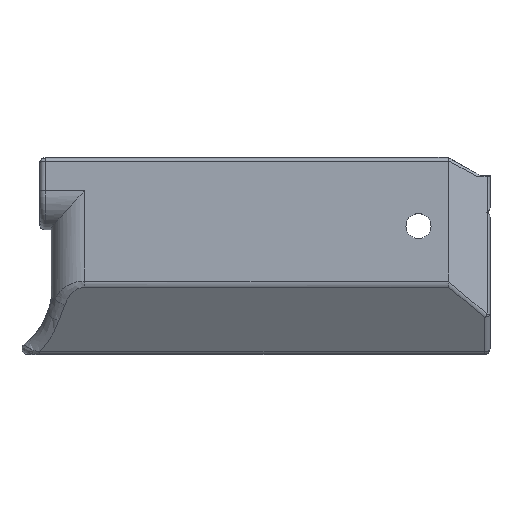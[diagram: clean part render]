
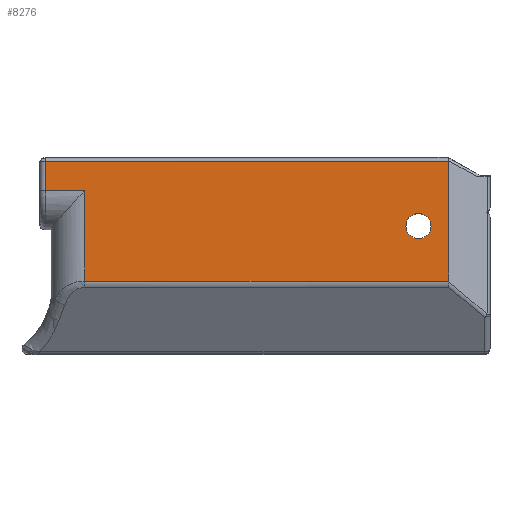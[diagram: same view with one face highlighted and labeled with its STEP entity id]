
A CAD part, top view. The second image highlights one B-rep face of the part: STEP entity #8276.
In plain terms, the highlighted planar face has unit normal (0, 0, 1).
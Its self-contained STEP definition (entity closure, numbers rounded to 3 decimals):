
#42=FACE_BOUND('',#2025,.T.);
#1062=PLANE('',#8491);
#1556=FACE_OUTER_BOUND('',#2024,.T.);
#2024=EDGE_LOOP('',(#7696,#7697,#7698,#7699,#7700,#7701));
#2025=EDGE_LOOP('',(#7702));
#2065=LINE('',#9587,#2628);
#2071=LINE('',#9659,#2634);
#2587=LINE('',#16405,#3150);
#2588=LINE('',#16408,#3151);
#2589=LINE('',#16409,#3152);
#2590=LINE('',#16410,#3153);
#2628=VECTOR('',#8560,10.);
#2634=VECTOR('',#8594,10.);
#3150=VECTOR('',#9428,10.);
#3151=VECTOR('',#9431,7.);
#3152=VECTOR('',#9432,10.);
#3153=VECTOR('',#9433,10.);
#3197=CIRCLE('',#8425,2.25);
#3244=VERTEX_POINT('',#9584);
#3245=VERTEX_POINT('',#9586);
#3255=VERTEX_POINT('',#9657);
#3990=VERTEX_POINT('',#15801);
#4042=VERTEX_POINT('',#16399);
#4043=VERTEX_POINT('',#16403);
#4044=VERTEX_POINT('',#16407);
#4079=EDGE_CURVE('',#3244,#3245,#2065,.T.);
#4095=EDGE_CURVE('',#3255,#3244,#2071,.T.);
#5192=EDGE_CURVE('',#3990,#3990,#3197,.T.);
#5281=EDGE_CURVE('',#4043,#4042,#2587,.T.);
#5282=EDGE_CURVE('',#4044,#3255,#2588,.T.);
#5283=EDGE_CURVE('',#4042,#4044,#2589,.T.);
#5284=EDGE_CURVE('',#4043,#3245,#2590,.T.);
#7696=ORIENTED_EDGE('',*,*,#4079,.F.);
#7697=ORIENTED_EDGE('',*,*,#4095,.F.);
#7698=ORIENTED_EDGE('',*,*,#5282,.F.);
#7699=ORIENTED_EDGE('',*,*,#5283,.F.);
#7700=ORIENTED_EDGE('',*,*,#5281,.F.);
#7701=ORIENTED_EDGE('',*,*,#5284,.T.);
#7702=ORIENTED_EDGE('',*,*,#5192,.F.);
#8276=ADVANCED_FACE('',(#1556,#42),#1062,.T.);
#8425=AXIS2_PLACEMENT_3D('',#15803,#9263,#9264);
#8491=AXIS2_PLACEMENT_3D('',#16406,#9429,#9430);
#8560=DIRECTION('',(1.,0.,0.));
#8594=DIRECTION('',(0.,1.,0.));
#9263=DIRECTION('center_axis',(0.,0.,1.));
#9264=DIRECTION('ref_axis',(-1.,0.,0.));
#9428=DIRECTION('',(-1.,0.,0.));
#9429=DIRECTION('center_axis',(0.,0.,1.));
#9430=DIRECTION('ref_axis',(0.,1.,0.));
#9431=DIRECTION('',(-1.,0.,0.));
#9432=DIRECTION('',(0.,1.,0.));
#9433=DIRECTION('',(0.,1.,0.));
#9584=CARTESIAN_POINT('',(39.384,39.543,-5.001));
#9586=CARTESIAN_POINT('',(111.609,39.543,-5.001));
#9587=CARTESIAN_POINT('',(119.034,39.543,-5.001));
#9657=CARTESIAN_POINT('',(39.384,34.251,-5.001));
#9659=CARTESIAN_POINT('',(39.384,21.441,-5.001));
#15801=CARTESIAN_POINT('',(108.479,27.904,-5.001));
#15803=CARTESIAN_POINT('Origin',(106.229,27.904,-5.001));
#16399=CARTESIAN_POINT('',(46.442,18.058,-5.001));
#16403=CARTESIAN_POINT('',(111.609,18.058,-5.001));
#16405=CARTESIAN_POINT('',(119.034,18.058,-5.001));
#16406=CARTESIAN_POINT('Origin',(119.034,14.941,-5.001));
#16407=CARTESIAN_POINT('',(46.442,34.251,-5.001));
#16408=CARTESIAN_POINT('',(39.413,34.251,-5.001));
#16409=CARTESIAN_POINT('',(46.442,23.575,-5.001));
#16410=CARTESIAN_POINT('',(111.609,14.941,-5.001));
